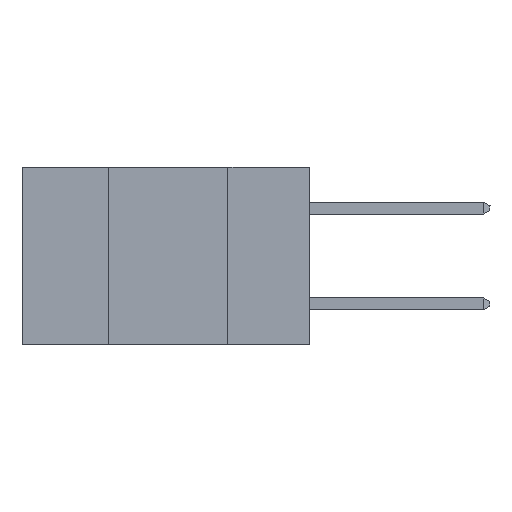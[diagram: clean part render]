
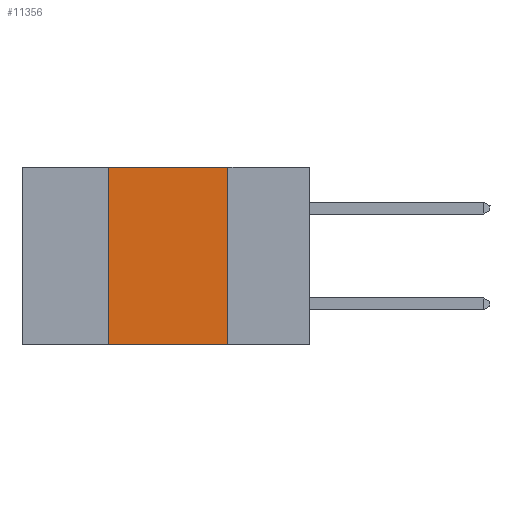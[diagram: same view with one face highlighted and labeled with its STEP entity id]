
A CAD part, left-side view. The second image highlights one B-rep face of the part: STEP entity #11356.
In plain terms, the highlighted planar face has unit normal (-1, 0, 0).
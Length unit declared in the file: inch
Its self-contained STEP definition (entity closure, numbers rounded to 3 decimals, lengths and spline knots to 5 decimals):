
#145 = VECTOR ( 'NONE', #7579, 39.37008 ) ;
#2702 = ORIENTED_EDGE ( 'NONE', *, *, #6024, .F. ) ;
#2781 = DIRECTION ( 'NONE',  ( 0., -1., 0. ) ) ;
#4194 = EDGE_CURVE ( 'NONE', #10389, #25510, #24461, .T. ) ;
#5219 = DIRECTION ( 'NONE',  ( 1., 0., 0. ) ) ;
#5263 = ORIENTED_EDGE ( 'NONE', *, *, #4194, .F. ) ;
#5616 = VECTOR ( 'NONE', #2781, 39.37008 ) ;
#6024 = EDGE_CURVE ( 'NONE', #12341, #10389, #24353, .T. ) ;
#7542 = DIRECTION ( 'NONE',  ( 0., -1., 0. ) ) ;
#7579 = DIRECTION ( 'NONE',  ( 0., 0., -1. ) ) ;
#7959 = EDGE_CURVE ( 'NONE', #19851, #25510, #17674, .T. ) ;
#8579 = CARTESIAN_POINT ( 'NONE',  ( 0., 0.42, 0. ) ) ;
#9825 = CARTESIAN_POINT ( 'NONE',  ( 0., 0.17, 0. ) ) ;
#10389 = VERTEX_POINT ( 'NONE', #11575 ) ;
#11356 = ADVANCED_FACE ( 'NONE', ( #24369 ), #16931, .F. ) ;
#11575 = CARTESIAN_POINT ( 'NONE',  ( 0., 0.17, 0. ) ) ;
#11676 = EDGE_LOOP ( 'NONE', ( #5263, #2702, #25458, #29055 ) ) ;
#12341 = VERTEX_POINT ( 'NONE', #8579 ) ;
#14498 = CARTESIAN_POINT ( 'NONE',  ( 0., 0.6, -0.37 ) ) ;
#15423 = VECTOR ( 'NONE', #24970, 39.37008 ) ;
#15781 = CARTESIAN_POINT ( 'NONE',  ( 0., 0.17, -0.37 ) ) ;
#16161 = LINE ( 'NONE', #27289, #15423 ) ;
#16931 = PLANE ( 'NONE',  #18535 ) ;
#17674 = LINE ( 'NONE', #14498, #27907 ) ;
#18535 = AXIS2_PLACEMENT_3D ( 'NONE', #21550, #5219, #21652 ) ;
#19255 = CARTESIAN_POINT ( 'NONE',  ( 0., 0.6, 0. ) ) ;
#19851 = VERTEX_POINT ( 'NONE', #27543 ) ;
#21550 = CARTESIAN_POINT ( 'NONE',  ( 0., 0.6, 0. ) ) ;
#21652 = DIRECTION ( 'NONE',  ( 0., 0., -1. ) ) ;
#24353 = LINE ( 'NONE', #19255, #5616 ) ;
#24369 = FACE_OUTER_BOUND ( 'NONE', #11676, .T. ) ;
#24461 = LINE ( 'NONE', #9825, #145 ) ;
#24970 = DIRECTION ( 'NONE',  ( 0., 0., 1. ) ) ;
#25458 = ORIENTED_EDGE ( 'NONE', *, *, #26792, .F. ) ;
#25510 = VERTEX_POINT ( 'NONE', #15781 ) ;
#26792 = EDGE_CURVE ( 'NONE', #19851, #12341, #16161, .T. ) ;
#27289 = CARTESIAN_POINT ( 'NONE',  ( 0., 0.42, 0. ) ) ;
#27543 = CARTESIAN_POINT ( 'NONE',  ( 0., 0.42, -0.37 ) ) ;
#27907 = VECTOR ( 'NONE', #7542, 39.37008 ) ;
#29055 = ORIENTED_EDGE ( 'NONE', *, *, #7959, .T. ) ;
